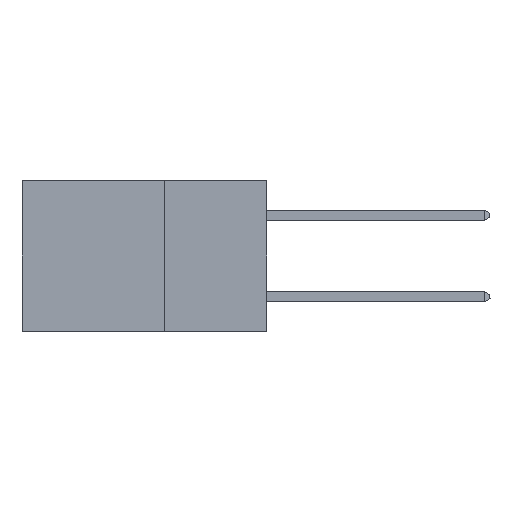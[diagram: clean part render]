
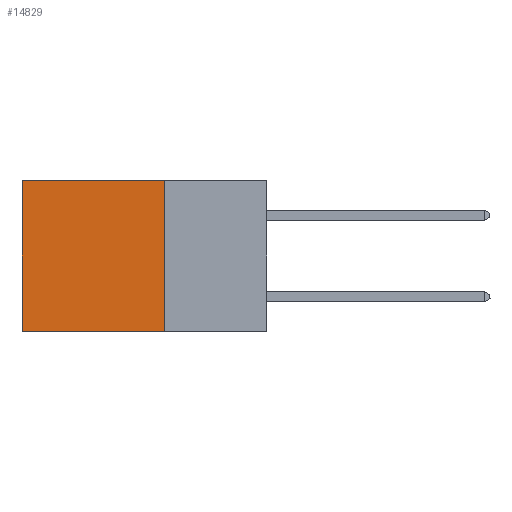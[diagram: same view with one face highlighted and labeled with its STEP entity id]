
A CAD part, left-side view. The second image highlights one B-rep face of the part: STEP entity #14829.
In plain terms, the highlighted planar face has unit normal (-1, 0, 0).
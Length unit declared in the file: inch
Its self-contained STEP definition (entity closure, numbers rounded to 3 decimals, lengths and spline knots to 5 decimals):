
#82 = FACE_OUTER_BOUND ( 'NONE', #16552, .T. ) ;
#3076 = CARTESIAN_POINT ( 'NONE',  ( 0.2875, 0.25, 0. ) ) ;
#3262 = DIRECTION ( 'NONE',  ( 0., 1., 0. ) ) ;
#3891 = DIRECTION ( 'NONE',  ( 0., 0., -1. ) ) ;
#3918 = VERTEX_POINT ( 'NONE', #18001 ) ;
#4790 = ORIENTED_EDGE ( 'NONE', *, *, #13304, .T. ) ;
#4974 = EDGE_CURVE ( 'NONE', #17483, #12637, #22661, .T. ) ;
#5040 = CARTESIAN_POINT ( 'NONE',  ( 0.2875, 0.25, 0. ) ) ;
#6091 = ORIENTED_EDGE ( 'NONE', *, *, #4974, .F. ) ;
#6263 = PLANE ( 'NONE',  #10978 ) ;
#6982 = DIRECTION ( 'NONE',  ( 1., 0., 0. ) ) ;
#7285 = EDGE_CURVE ( 'NONE', #16987, #17483, #17752, .T. ) ;
#7345 = VECTOR ( 'NONE', #3891, 39.37008 ) ;
#7652 = CARTESIAN_POINT ( 'NONE',  ( 0.2875, 0.25, 0. ) ) ;
#8480 = ORIENTED_EDGE ( 'NONE', *, *, #20409, .T. ) ;
#8935 = CARTESIAN_POINT ( 'NONE',  ( 0.2875, 0.25, -0.37 ) ) ;
#9960 = CARTESIAN_POINT ( 'NONE',  ( 0.2875, 0.6, 0. ) ) ;
#10436 = CARTESIAN_POINT ( 'NONE',  ( 0.2875, 0.25, 0. ) ) ;
#10978 = AXIS2_PLACEMENT_3D ( 'NONE', #10436, #6982, #11157 ) ;
#11157 = DIRECTION ( 'NONE',  ( 0., 0., -1. ) ) ;
#11333 = VECTOR ( 'NONE', #14057, 39.37008 ) ;
#11601 = ORIENTED_EDGE ( 'NONE', *, *, #7285, .F. ) ;
#12637 = VERTEX_POINT ( 'NONE', #19461 ) ;
#13304 = EDGE_CURVE ( 'NONE', #16987, #3918, #25485, .T. ) ;
#14057 = DIRECTION ( 'NONE',  ( 0., 1., 0. ) ) ;
#14829 = ADVANCED_FACE ( 'NONE', ( #82 ), #6263, .F. ) ;
#15237 = CARTESIAN_POINT ( 'NONE',  ( 0.2875, 0.25, -0.37 ) ) ;
#16552 = EDGE_LOOP ( 'NONE', ( #8480, #6091, #11601, #4790 ) ) ;
#16987 = VERTEX_POINT ( 'NONE', #5040 ) ;
#17483 = VERTEX_POINT ( 'NONE', #15237 ) ;
#17645 = LINE ( 'NONE', #9960, #7345 ) ;
#17752 = LINE ( 'NONE', #3076, #21921 ) ;
#18001 = CARTESIAN_POINT ( 'NONE',  ( 0.2875, 0.6, 0. ) ) ;
#19461 = CARTESIAN_POINT ( 'NONE',  ( 0.2875, 0.6, -0.37 ) ) ;
#20409 = EDGE_CURVE ( 'NONE', #3918, #12637, #17645, .T. ) ;
#20894 = VECTOR ( 'NONE', #3262, 39.37008 ) ;
#21921 = VECTOR ( 'NONE', #23334, 39.37008 ) ;
#22661 = LINE ( 'NONE', #8935, #20894 ) ;
#23334 = DIRECTION ( 'NONE',  ( 0., 0., -1. ) ) ;
#25485 = LINE ( 'NONE', #7652, #11333 ) ;
